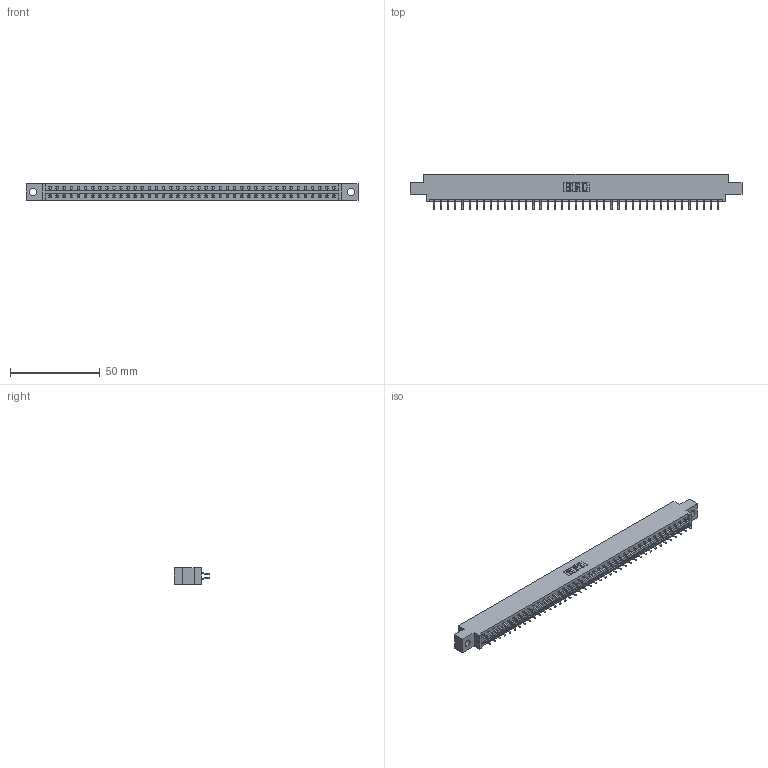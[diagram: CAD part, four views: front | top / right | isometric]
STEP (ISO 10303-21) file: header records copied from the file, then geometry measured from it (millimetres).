
FILE_DESCRIPTION (( 'STEP AP203' ), '1' );
FILE_NAME ('387-082-556-804.STEP', '2019-10-23T00:17:27', ( '' ), ( '' ), 'SwSTEP 2.0', 'SolidWorks 2016', '' );
FILE_SCHEMA (( 'CONFIG_CONTROL_DESIGN' ));
Length unit declared in the file: inch
Products named in the file (3): 387-082-556-804; 345-292-001_556 Tail; 337 Part_0.170 Offset - 0.156 Dia-TH
Assembly tree (83 placements, depth 2):
  387-082-556-804
    337 Part_0.170 Offset - 0.156 Dia-TH
    345-292-001_556 Tail  x82
Bounding box: 185.47 x 19.57 x 9.4 mm (x, y, z)
Volume: 19324.5 mm3; surface area: 21655.3 mm2
Topology: 83 solids, 83 shells, 5038 faces, 15001 edges, 9890 vertices
Faces by surface type: plane 3518, cylinder 1520
Entity records: 32273 total; most frequent: CARTESIAN_POINT 5454, ORIENTED_EDGE 5378, DIRECTION 4629, EDGE_CURVE 2689, LINE 2553, VECTOR 2553, VERTEX_POINT 1790, AXIS2_PLACEMENT_3D 1038
